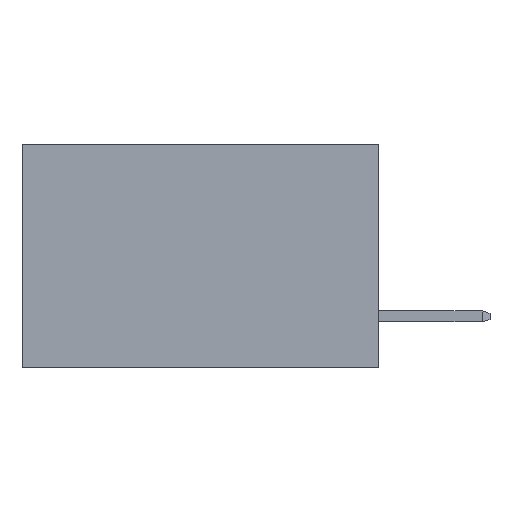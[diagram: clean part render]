
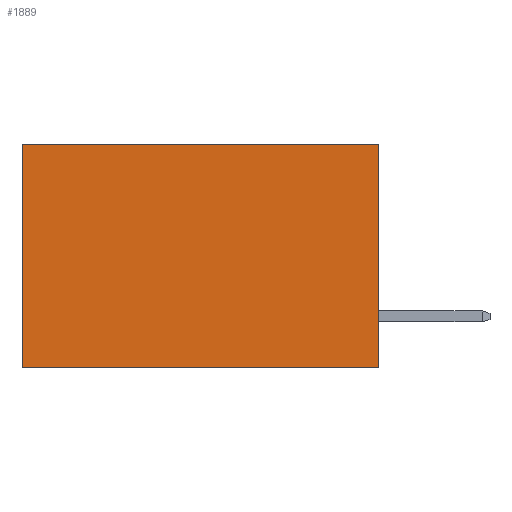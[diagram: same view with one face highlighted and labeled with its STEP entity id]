
A CAD part, left-side view. The second image highlights one B-rep face of the part: STEP entity #1889.
In plain terms, the highlighted planar face has unit normal (-1, 0, 0).
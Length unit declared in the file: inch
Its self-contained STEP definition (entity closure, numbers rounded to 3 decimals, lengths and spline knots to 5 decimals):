
#592 = CARTESIAN_POINT ( 'NONE',  ( 0.277, 0., -0.37 ) ) ;
#597 = VECTOR ( 'NONE', #2596, 39.37008 ) ;
#996 = PLANE ( 'NONE',  #3850 ) ;
#1042 = FACE_OUTER_BOUND ( 'NONE', #1270, .T. ) ;
#1166 = EDGE_CURVE ( 'NONE', #7893, #4671, #3631, .T. ) ;
#1270 = EDGE_LOOP ( 'NONE', ( #6244, #6426, #6503, #6837 ) ) ;
#1713 = CARTESIAN_POINT ( 'NONE',  ( 0.277, 0., -0.37 ) ) ;
#1889 = ADVANCED_FACE ( 'NONE', ( #1042 ), #996, .F. ) ;
#1923 = EDGE_CURVE ( 'NONE', #4671, #3919, #4853, .T. ) ;
#2044 = EDGE_CURVE ( 'NONE', #4576, #3919, #8063, .T. ) ;
#2204 = DIRECTION ( 'NONE',  ( 0., 1., 0. ) ) ;
#2336 = DIRECTION ( 'NONE',  ( 0., 0., -1. ) ) ;
#2596 = DIRECTION ( 'NONE',  ( 0., 0., -1. ) ) ;
#2747 = VECTOR ( 'NONE', #2336, 39.37008 ) ;
#3318 = DIRECTION ( 'NONE',  ( 0., 0., -1. ) ) ;
#3330 = CARTESIAN_POINT ( 'NONE',  ( 0.277, 0., 0. ) ) ;
#3498 = CARTESIAN_POINT ( 'NONE',  ( 0.277, 0., -0.37 ) ) ;
#3631 = LINE ( 'NONE', #8874, #9360 ) ;
#3850 = AXIS2_PLACEMENT_3D ( 'NONE', #3498, #8593, #3318 ) ;
#3919 = VERTEX_POINT ( 'NONE', #6455 ) ;
#4576 = VERTEX_POINT ( 'NONE', #7011 ) ;
#4671 = VERTEX_POINT ( 'NONE', #6597 ) ;
#4853 = LINE ( 'NONE', #4960, #2747 ) ;
#4916 = LINE ( 'NONE', #1713, #597 ) ;
#4960 = CARTESIAN_POINT ( 'NONE',  ( 0.277, 0.59, -0.37 ) ) ;
#6244 = ORIENTED_EDGE ( 'NONE', *, *, #1923, .T. ) ;
#6426 = ORIENTED_EDGE ( 'NONE', *, *, #2044, .F. ) ;
#6455 = CARTESIAN_POINT ( 'NONE',  ( 0.277, 0.59, -0.37 ) ) ;
#6503 = ORIENTED_EDGE ( 'NONE', *, *, #9843, .F. ) ;
#6597 = CARTESIAN_POINT ( 'NONE',  ( 0.277, 0.59, 0. ) ) ;
#6837 = ORIENTED_EDGE ( 'NONE', *, *, #1166, .T. ) ;
#7011 = CARTESIAN_POINT ( 'NONE',  ( 0.277, 0., -0.37 ) ) ;
#7893 = VERTEX_POINT ( 'NONE', #3330 ) ;
#8063 = LINE ( 'NONE', #592, #9760 ) ;
#8593 = DIRECTION ( 'NONE',  ( 1., 0., 0. ) ) ;
#8791 = DIRECTION ( 'NONE',  ( 0., 1., 0. ) ) ;
#8874 = CARTESIAN_POINT ( 'NONE',  ( 0.277, 0., 0. ) ) ;
#9360 = VECTOR ( 'NONE', #8791, 39.37008 ) ;
#9760 = VECTOR ( 'NONE', #2204, 39.37008 ) ;
#9843 = EDGE_CURVE ( 'NONE', #7893, #4576, #4916, .T. ) ;
